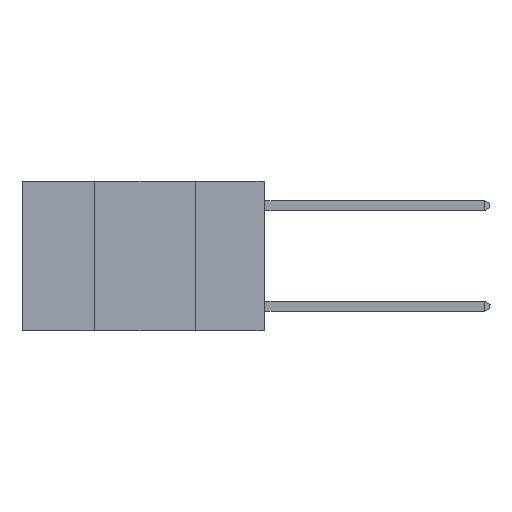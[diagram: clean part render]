
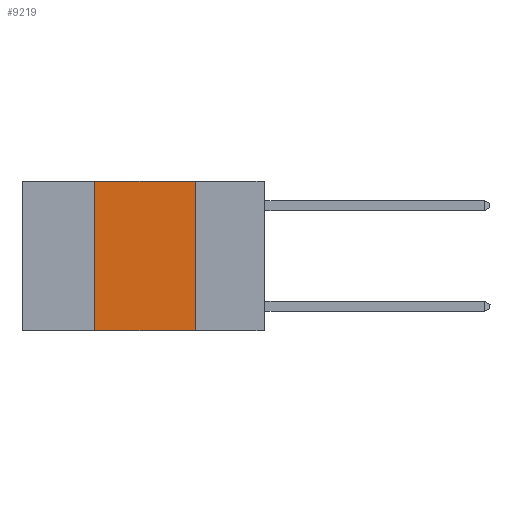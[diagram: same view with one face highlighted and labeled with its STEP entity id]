
A CAD part, left-side view. The second image highlights one B-rep face of the part: STEP entity #9219.
In plain terms, the highlighted planar face has unit normal (-1, 0, 0).
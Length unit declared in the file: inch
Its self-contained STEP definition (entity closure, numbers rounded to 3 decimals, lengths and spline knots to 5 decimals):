
#461 = ORIENTED_EDGE ( 'NONE', *, *, #8494, .F. ) ;
#646 = VECTOR ( 'NONE', #2938, 39.37008 ) ;
#699 = ORIENTED_EDGE ( 'NONE', *, *, #5711, .F. ) ;
#898 = ORIENTED_EDGE ( 'NONE', *, *, #16765, .T. ) ;
#935 = ORIENTED_EDGE ( 'NONE', *, *, #2561, .F. ) ;
#1024 = VERTEX_POINT ( 'NONE', #3438 ) ;
#1520 = VECTOR ( 'NONE', #13031, 39.37008 ) ;
#1685 = VECTOR ( 'NONE', #4615, 39.37008 ) ;
#2408 = VECTOR ( 'NONE', #9958, 39.37008 ) ;
#2561 = EDGE_CURVE ( 'NONE', #12371, #1024, #5063, .T. ) ;
#2938 = DIRECTION ( 'NONE',  ( 0., -1., 0. ) ) ;
#3176 = CARTESIAN_POINT ( 'NONE',  ( 0., 0.42, 0. ) ) ;
#3313 = LINE ( 'NONE', #3176, #2408 ) ;
#3438 = CARTESIAN_POINT ( 'NONE',  ( 0., 0.17, -0.37 ) ) ;
#3478 = AXIS2_PLACEMENT_3D ( 'NONE', #10895, #13674, #5619 ) ;
#3571 = CARTESIAN_POINT ( 'NONE',  ( 0., 0.6, -0.37 ) ) ;
#4102 = LINE ( 'NONE', #11028, #646 ) ;
#4615 = DIRECTION ( 'NONE',  ( 0., 0., -1. ) ) ;
#4957 = VERTEX_POINT ( 'NONE', #5264 ) ;
#5063 = LINE ( 'NONE', #11289, #1685 ) ;
#5264 = CARTESIAN_POINT ( 'NONE',  ( 0., 0.42, -0.37 ) ) ;
#5336 = LINE ( 'NONE', #3571, #1520 ) ;
#5537 = CARTESIAN_POINT ( 'NONE',  ( 0., 0.17, 0. ) ) ;
#5560 = PLANE ( 'NONE',  #3478 ) ;
#5619 = DIRECTION ( 'NONE',  ( 0., 0., -1. ) ) ;
#5711 = EDGE_CURVE ( 'NONE', #4957, #6222, #3313, .T. ) ;
#6222 = VERTEX_POINT ( 'NONE', #8289 ) ;
#8289 = CARTESIAN_POINT ( 'NONE',  ( 0., 0.42, 0. ) ) ;
#8494 = EDGE_CURVE ( 'NONE', #6222, #12371, #4102, .T. ) ;
#9063 = EDGE_LOOP ( 'NONE', ( #935, #461, #699, #898 ) ) ;
#9219 = ADVANCED_FACE ( 'NONE', ( #13169 ), #5560, .F. ) ;
#9958 = DIRECTION ( 'NONE',  ( 0., 0., 1. ) ) ;
#10895 = CARTESIAN_POINT ( 'NONE',  ( 0., 0.6, 0. ) ) ;
#11028 = CARTESIAN_POINT ( 'NONE',  ( 0., 0.6, 0. ) ) ;
#11289 = CARTESIAN_POINT ( 'NONE',  ( 0., 0.17, 0. ) ) ;
#12371 = VERTEX_POINT ( 'NONE', #5537 ) ;
#13031 = DIRECTION ( 'NONE',  ( 0., -1., 0. ) ) ;
#13169 = FACE_OUTER_BOUND ( 'NONE', #9063, .T. ) ;
#13674 = DIRECTION ( 'NONE',  ( 1., 0., 0. ) ) ;
#16765 = EDGE_CURVE ( 'NONE', #4957, #1024, #5336, .T. ) ;
